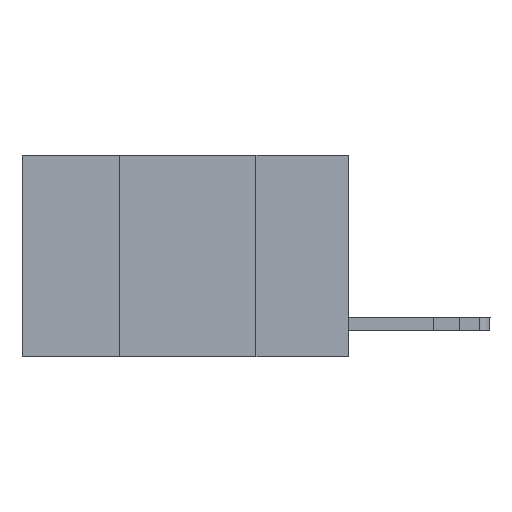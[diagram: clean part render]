
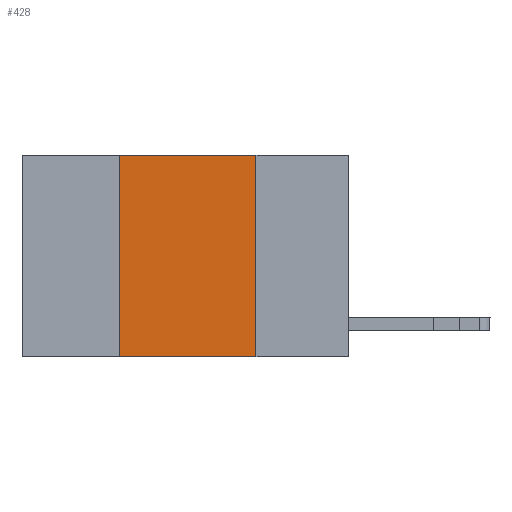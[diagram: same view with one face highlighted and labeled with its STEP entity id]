
A CAD part, left-side view. The second image highlights one B-rep face of the part: STEP entity #428.
In plain terms, the highlighted planar face has unit normal (-1, 0, 0).
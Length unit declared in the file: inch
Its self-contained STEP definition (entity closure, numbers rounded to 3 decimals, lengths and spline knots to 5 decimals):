
#428 = ADVANCED_FACE ( 'NONE', ( #6845 ), #572, .F. ) ;
#572 = PLANE ( 'NONE',  #7729 ) ;
#670 = DIRECTION ( 'NONE',  ( 0., 0., -1. ) ) ;
#1821 = EDGE_CURVE ( 'NONE', #14477, #4186, #16291, .T. ) ;
#2839 = CARTESIAN_POINT ( 'NONE',  ( 0., 0.17, 0. ) ) ;
#3202 = CARTESIAN_POINT ( 'NONE',  ( 0., 0.17, -0.37 ) ) ;
#3952 = DIRECTION ( 'NONE',  ( 0., 0., 1. ) ) ;
#4186 = VERTEX_POINT ( 'NONE', #3202 ) ;
#4483 = DIRECTION ( 'NONE',  ( 0., 0., -1. ) ) ;
#5710 = VECTOR ( 'NONE', #15514, 39.37008 ) ;
#6083 = EDGE_LOOP ( 'NONE', ( #18960, #10172, #19864, #6871 ) ) ;
#6845 = FACE_OUTER_BOUND ( 'NONE', #6083, .T. ) ;
#6871 = ORIENTED_EDGE ( 'NONE', *, *, #1821, .T. ) ;
#7541 = VECTOR ( 'NONE', #12376, 39.37008 ) ;
#7729 = AXIS2_PLACEMENT_3D ( 'NONE', #14859, #14817, #670 ) ;
#9431 = VERTEX_POINT ( 'NONE', #19042 ) ;
#10112 = LINE ( 'NONE', #17077, #5710 ) ;
#10172 = ORIENTED_EDGE ( 'NONE', *, *, #14650, .F. ) ;
#10426 = CARTESIAN_POINT ( 'NONE',  ( 0., 0.42, 0. ) ) ;
#10460 = LINE ( 'NONE', #2839, #18571 ) ;
#12325 = CARTESIAN_POINT ( 'NONE',  ( 0., 0.6, -0.37 ) ) ;
#12376 = DIRECTION ( 'NONE',  ( 0., -1., 0. ) ) ;
#13993 = VECTOR ( 'NONE', #3952, 39.37008 ) ;
#14477 = VERTEX_POINT ( 'NONE', #20672 ) ;
#14650 = EDGE_CURVE ( 'NONE', #18242, #9431, #10112, .T. ) ;
#14817 = DIRECTION ( 'NONE',  ( 1., 0., 0. ) ) ;
#14859 = CARTESIAN_POINT ( 'NONE',  ( 0., 0.6, 0. ) ) ;
#15514 = DIRECTION ( 'NONE',  ( 0., -1., 0. ) ) ;
#16291 = LINE ( 'NONE', #12325, #7541 ) ;
#17077 = CARTESIAN_POINT ( 'NONE',  ( 0., 0.6, 0. ) ) ;
#17857 = CARTESIAN_POINT ( 'NONE',  ( 0., 0.42, 0. ) ) ;
#18242 = VERTEX_POINT ( 'NONE', #17857 ) ;
#18280 = LINE ( 'NONE', #10426, #13993 ) ;
#18571 = VECTOR ( 'NONE', #4483, 39.37008 ) ;
#18641 = EDGE_CURVE ( 'NONE', #9431, #4186, #10460, .T. ) ;
#18960 = ORIENTED_EDGE ( 'NONE', *, *, #18641, .F. ) ;
#19042 = CARTESIAN_POINT ( 'NONE',  ( 0., 0.17, 0. ) ) ;
#19737 = EDGE_CURVE ( 'NONE', #14477, #18242, #18280, .T. ) ;
#19864 = ORIENTED_EDGE ( 'NONE', *, *, #19737, .F. ) ;
#20672 = CARTESIAN_POINT ( 'NONE',  ( 0., 0.42, -0.37 ) ) ;
